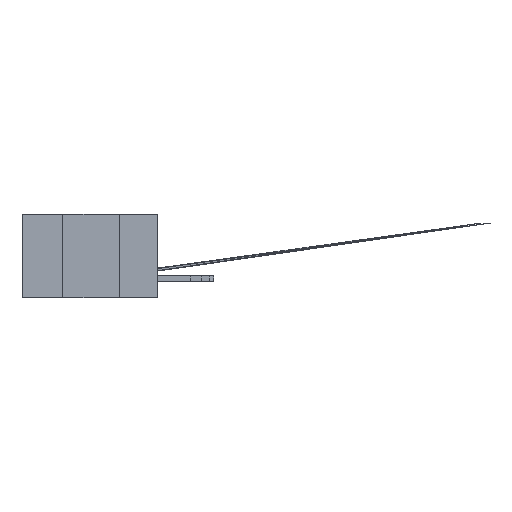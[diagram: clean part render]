
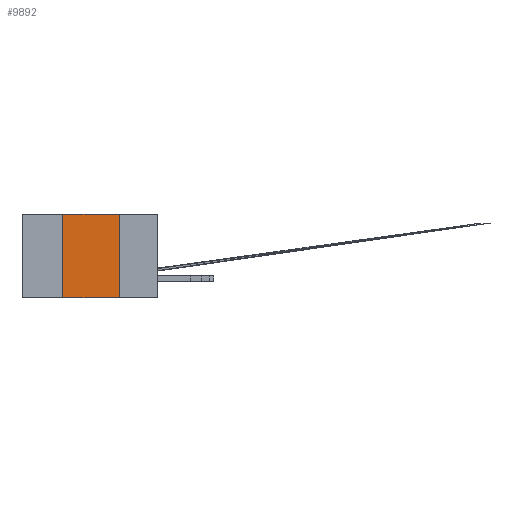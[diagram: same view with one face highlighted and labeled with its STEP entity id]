
A CAD part, left-side view. The second image highlights one B-rep face of the part: STEP entity #9892.
In plain terms, the highlighted planar face has unit normal (-1, 0, 0).
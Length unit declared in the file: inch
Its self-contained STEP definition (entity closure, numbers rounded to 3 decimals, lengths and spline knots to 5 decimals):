
#634 = LINE ( 'NONE', #4501, #7525 ) ;
#646 = EDGE_CURVE ( 'NONE', #8914, #3863, #3764, .T. ) ;
#1192 = DIRECTION ( 'NONE',  ( 0., 0., -1. ) ) ;
#1390 = ORIENTED_EDGE ( 'NONE', *, *, #3720, .T. ) ;
#1557 = CARTESIAN_POINT ( 'NONE',  ( 0., 0.42, -0.37 ) ) ;
#2036 = DIRECTION ( 'NONE',  ( 1., 0., 0. ) ) ;
#2837 = VERTEX_POINT ( 'NONE', #1557 ) ;
#3167 = FACE_OUTER_BOUND ( 'NONE', #3637, .T. ) ;
#3336 = ORIENTED_EDGE ( 'NONE', *, *, #5495, .F. ) ;
#3346 = VECTOR ( 'NONE', #1192, 39.37008 ) ;
#3637 = EDGE_LOOP ( 'NONE', ( #3652, #14689, #3336, #1390 ) ) ;
#3652 = ORIENTED_EDGE ( 'NONE', *, *, #646, .F. ) ;
#3720 = EDGE_CURVE ( 'NONE', #2837, #3863, #12960, .T. ) ;
#3764 = LINE ( 'NONE', #15866, #3346 ) ;
#3863 = VERTEX_POINT ( 'NONE', #8566 ) ;
#4440 = DIRECTION ( 'NONE',  ( 0., -1., 0. ) ) ;
#4501 = CARTESIAN_POINT ( 'NONE',  ( 0., 0.6, 0. ) ) ;
#5495 = EDGE_CURVE ( 'NONE', #2837, #10179, #11543, .T. ) ;
#5760 = EDGE_CURVE ( 'NONE', #10179, #8914, #634, .T. ) ;
#7525 = VECTOR ( 'NONE', #4440, 39.37008 ) ;
#8155 = VECTOR ( 'NONE', #14532, 39.37008 ) ;
#8566 = CARTESIAN_POINT ( 'NONE',  ( 0., 0.17, -0.37 ) ) ;
#8914 = VERTEX_POINT ( 'NONE', #15306 ) ;
#9892 = ADVANCED_FACE ( 'NONE', ( #3167 ), #11248, .F. ) ;
#10048 = CARTESIAN_POINT ( 'NONE',  ( 0., 0.6, 0. ) ) ;
#10179 = VERTEX_POINT ( 'NONE', #15523 ) ;
#11248 = PLANE ( 'NONE',  #11249 ) ;
#11249 = AXIS2_PLACEMENT_3D ( 'NONE', #10048, #2036, #11297 ) ;
#11297 = DIRECTION ( 'NONE',  ( 0., 0., -1. ) ) ;
#11543 = LINE ( 'NONE', #14675, #8155 ) ;
#11577 = CARTESIAN_POINT ( 'NONE',  ( 0., 0.6, -0.37 ) ) ;
#11626 = DIRECTION ( 'NONE',  ( 0., -1., 0. ) ) ;
#12213 = VECTOR ( 'NONE', #11626, 39.37008 ) ;
#12960 = LINE ( 'NONE', #11577, #12213 ) ;
#14532 = DIRECTION ( 'NONE',  ( 0., 0., 1. ) ) ;
#14675 = CARTESIAN_POINT ( 'NONE',  ( 0., 0.42, 0. ) ) ;
#14689 = ORIENTED_EDGE ( 'NONE', *, *, #5760, .F. ) ;
#15306 = CARTESIAN_POINT ( 'NONE',  ( 0., 0.17, 0. ) ) ;
#15523 = CARTESIAN_POINT ( 'NONE',  ( 0., 0.42, 0. ) ) ;
#15866 = CARTESIAN_POINT ( 'NONE',  ( 0., 0.17, 0. ) ) ;
